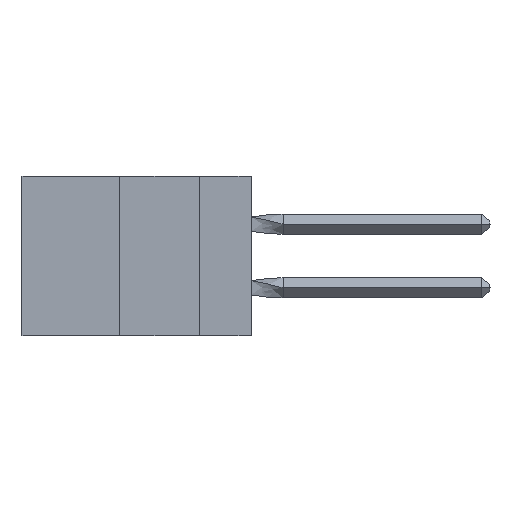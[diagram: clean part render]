
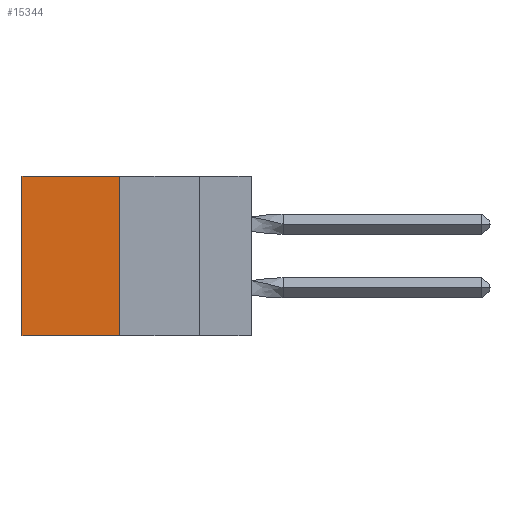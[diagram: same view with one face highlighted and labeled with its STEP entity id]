
A CAD part, left-side view. The second image highlights one B-rep face of the part: STEP entity #15344.
In plain terms, the highlighted planar face has unit normal (-1, 0, 0).
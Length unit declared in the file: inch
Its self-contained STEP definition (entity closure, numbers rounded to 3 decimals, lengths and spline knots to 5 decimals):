
#1782 = LINE ( 'NONE', #17406, #37096 ) ;
#2898 = DIRECTION ( 'NONE',  ( 0., 1., 0. ) ) ;
#5338 = LINE ( 'NONE', #17414, #37472 ) ;
#5363 = AXIS2_PLACEMENT_3D ( 'NONE', #6182, #12037, #20740 ) ;
#6182 = CARTESIAN_POINT ( 'NONE',  ( 0.305, 0.413, -0.5 ) ) ;
#6798 = DIRECTION ( 'NONE',  ( 0., 0., -1. ) ) ;
#7012 = VERTEX_POINT ( 'NONE', #12477 ) ;
#7213 = LINE ( 'NONE', #12784, #27137 ) ;
#12037 = DIRECTION ( 'NONE',  ( 1., 0., 0. ) ) ;
#12477 = CARTESIAN_POINT ( 'NONE',  ( 0.305, 0.72, -0.5 ) ) ;
#12784 = CARTESIAN_POINT ( 'NONE',  ( 0.305, 0.413, -0.5 ) ) ;
#12856 = LINE ( 'NONE', #29664, #23956 ) ;
#13812 = CARTESIAN_POINT ( 'NONE',  ( 0.305, 0.72, 0. ) ) ;
#14444 = ORIENTED_EDGE ( 'NONE', *, *, #38456, .F. ) ;
#15344 = ADVANCED_FACE ( 'NONE', ( #33741 ), #35708, .F. ) ;
#16939 = EDGE_LOOP ( 'NONE', ( #31811, #14444, #25059, #17233 ) ) ;
#17233 = ORIENTED_EDGE ( 'NONE', *, *, #37968, .T. ) ;
#17406 = CARTESIAN_POINT ( 'NONE',  ( 0.305, 0.72, -0.5 ) ) ;
#17414 = CARTESIAN_POINT ( 'NONE',  ( 0.305, 0.413, -0.5 ) ) ;
#20740 = DIRECTION ( 'NONE',  ( 0., 0., -1. ) ) ;
#21207 = CARTESIAN_POINT ( 'NONE',  ( 0.305, 0.413, 0. ) ) ;
#21770 = CARTESIAN_POINT ( 'NONE',  ( 0.305, 0.413, -0.5 ) ) ;
#21993 = VERTEX_POINT ( 'NONE', #21770 ) ;
#23633 = DIRECTION ( 'NONE',  ( 0., 1., 0. ) ) ;
#23956 = VECTOR ( 'NONE', #2898, 39.37008 ) ;
#24314 = VERTEX_POINT ( 'NONE', #21207 ) ;
#24719 = EDGE_CURVE ( 'NONE', #33076, #7012, #1782, .T. ) ;
#25059 = ORIENTED_EDGE ( 'NONE', *, *, #26223, .F. ) ;
#26223 = EDGE_CURVE ( 'NONE', #24314, #21993, #7213, .T. ) ;
#27137 = VECTOR ( 'NONE', #6798, 39.37008 ) ;
#29664 = CARTESIAN_POINT ( 'NONE',  ( 0.305, 0.413, 0. ) ) ;
#31811 = ORIENTED_EDGE ( 'NONE', *, *, #24719, .T. ) ;
#32233 = DIRECTION ( 'NONE',  ( 0., 0., -1. ) ) ;
#33076 = VERTEX_POINT ( 'NONE', #13812 ) ;
#33741 = FACE_OUTER_BOUND ( 'NONE', #16939, .T. ) ;
#35708 = PLANE ( 'NONE',  #5363 ) ;
#37096 = VECTOR ( 'NONE', #32233, 39.37008 ) ;
#37472 = VECTOR ( 'NONE', #23633, 39.37008 ) ;
#37968 = EDGE_CURVE ( 'NONE', #24314, #33076, #12856, .T. ) ;
#38456 = EDGE_CURVE ( 'NONE', #21993, #7012, #5338, .T. ) ;
